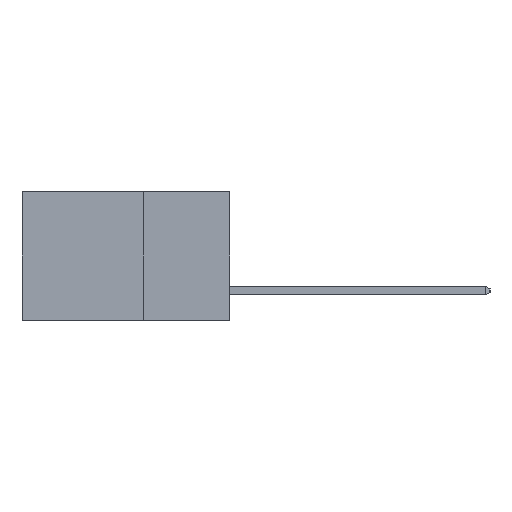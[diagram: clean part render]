
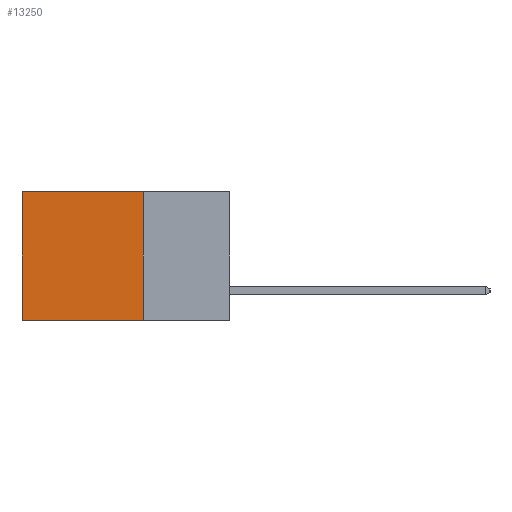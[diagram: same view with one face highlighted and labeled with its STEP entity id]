
A CAD part, left-side view. The second image highlights one B-rep face of the part: STEP entity #13250.
In plain terms, the highlighted planar face has unit normal (-1, 0, 0).
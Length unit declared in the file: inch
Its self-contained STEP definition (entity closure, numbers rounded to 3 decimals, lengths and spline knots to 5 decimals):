
#723 = LINE ( 'NONE', #12472, #14721 ) ;
#1439 = VERTEX_POINT ( 'NONE', #16617 ) ;
#2081 = DIRECTION ( 'NONE',  ( 0., 1., 0. ) ) ;
#2737 = VERTEX_POINT ( 'NONE', #9124 ) ;
#3529 = LINE ( 'NONE', #4707, #17424 ) ;
#4372 = CARTESIAN_POINT ( 'NONE',  ( 0.298, 0.25, 0. ) ) ;
#4707 = CARTESIAN_POINT ( 'NONE',  ( 0.298, 0.25, 0. ) ) ;
#6031 = ORIENTED_EDGE ( 'NONE', *, *, #20224, .F. ) ;
#8470 = CARTESIAN_POINT ( 'NONE',  ( 0.298, 0.6, 0. ) ) ;
#8659 = EDGE_CURVE ( 'NONE', #1439, #19071, #3529, .T. ) ;
#8685 = VECTOR ( 'NONE', #2081, 39.37008 ) ;
#9124 = CARTESIAN_POINT ( 'NONE',  ( 0.298, 0.6, -0.37 ) ) ;
#9767 = ORIENTED_EDGE ( 'NONE', *, *, #16299, .T. ) ;
#9833 = DIRECTION ( 'NONE',  ( 1., 0., 0. ) ) ;
#9984 = CARTESIAN_POINT ( 'NONE',  ( 0.298, 0.25, 0. ) ) ;
#10174 = ORIENTED_EDGE ( 'NONE', *, *, #15312, .T. ) ;
#11441 = FACE_OUTER_BOUND ( 'NONE', #17515, .T. ) ;
#12472 = CARTESIAN_POINT ( 'NONE',  ( 0.298, 0.6, 0. ) ) ;
#13198 = CARTESIAN_POINT ( 'NONE',  ( 0.298, 0.25, -0.37 ) ) ;
#13214 = LINE ( 'NONE', #21720, #8685 ) ;
#13250 = ADVANCED_FACE ( 'NONE', ( #11441 ), #18795, .F. ) ;
#14434 = ORIENTED_EDGE ( 'NONE', *, *, #8659, .F. ) ;
#14721 = VECTOR ( 'NONE', #17898, 39.37008 ) ;
#15312 = EDGE_CURVE ( 'NONE', #1439, #15406, #17579, .T. ) ;
#15406 = VERTEX_POINT ( 'NONE', #8470 ) ;
#16299 = EDGE_CURVE ( 'NONE', #15406, #2737, #723, .T. ) ;
#16617 = CARTESIAN_POINT ( 'NONE',  ( 0.298, 0.25, 0. ) ) ;
#17369 = DIRECTION ( 'NONE',  ( 0., 0., -1. ) ) ;
#17424 = VECTOR ( 'NONE', #17369, 39.37008 ) ;
#17515 = EDGE_LOOP ( 'NONE', ( #9767, #6031, #14434, #10174 ) ) ;
#17579 = LINE ( 'NONE', #9984, #21578 ) ;
#17898 = DIRECTION ( 'NONE',  ( 0., 0., -1. ) ) ;
#18795 = PLANE ( 'NONE',  #22765 ) ;
#19071 = VERTEX_POINT ( 'NONE', #13198 ) ;
#20224 = EDGE_CURVE ( 'NONE', #19071, #2737, #13214, .T. ) ;
#20631 = DIRECTION ( 'NONE',  ( 0., 1., 0. ) ) ;
#21578 = VECTOR ( 'NONE', #20631, 39.37008 ) ;
#21720 = CARTESIAN_POINT ( 'NONE',  ( 0.298, 0.25, -0.37 ) ) ;
#22228 = DIRECTION ( 'NONE',  ( 0., 0., -1. ) ) ;
#22765 = AXIS2_PLACEMENT_3D ( 'NONE', #4372, #9833, #22228 ) ;
